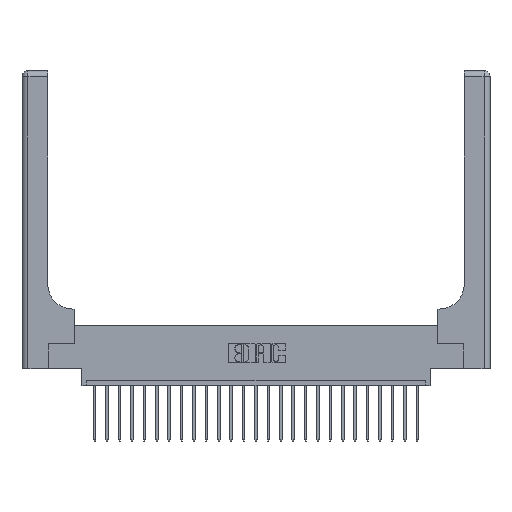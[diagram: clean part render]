
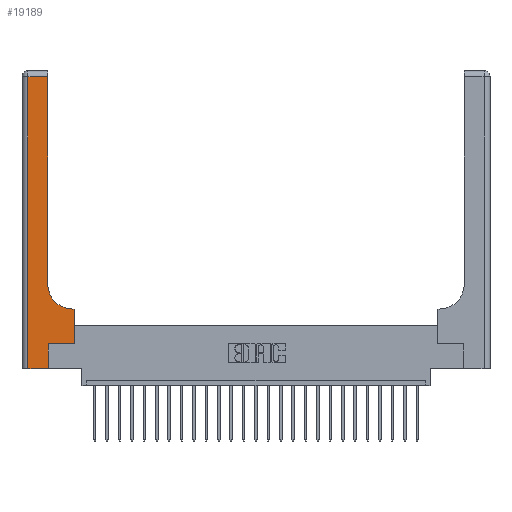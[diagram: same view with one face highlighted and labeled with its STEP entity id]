
A CAD part, top view. The second image highlights one B-rep face of the part: STEP entity #19189.
In plain terms, the highlighted planar face has unit normal (0, 0, 1).
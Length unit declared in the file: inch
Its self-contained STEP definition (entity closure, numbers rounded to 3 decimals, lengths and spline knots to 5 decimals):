
#389 = VERTEX_POINT ( 'NONE', #19670 ) ;
#482 = ORIENTED_EDGE ( 'NONE', *, *, #1757, .T. ) ;
#861 = AXIS2_PLACEMENT_3D ( 'NONE', #8938, #9064, #5103 ) ;
#1435 = DIRECTION ( 'NONE',  ( 1., 0., 0. ) ) ;
#1757 = EDGE_CURVE ( 'NONE', #12092, #18439, #12728, .T. ) ;
#1889 = CARTESIAN_POINT ( 'NONE',  ( 0.265, 0.25, 0.37 ) ) ;
#2095 = EDGE_CURVE ( 'NONE', #8628, #21289, #4739, .T. ) ;
#2150 = CARTESIAN_POINT ( 'NONE',  ( 0.528, 0.25, 0.37 ) ) ;
#2192 = AXIS2_PLACEMENT_3D ( 'NONE', #3518, #24505, #9337 ) ;
#2385 = ORIENTED_EDGE ( 'NONE', *, *, #19223, .T. ) ;
#3319 = CARTESIAN_POINT ( 'NONE',  ( 0.265, 0., 0.37 ) ) ;
#3518 = CARTESIAN_POINT ( 'NONE',  ( 0., 3., 0.37 ) ) ;
#3534 = CARTESIAN_POINT ( 'NONE',  ( 0.26, 3., 0.37 ) ) ;
#3911 = ORIENTED_EDGE ( 'NONE', *, *, #13607, .T. ) ;
#4010 = VECTOR ( 'NONE', #9216, 39.37008 ) ;
#4739 = LINE ( 'NONE', #19775, #7681 ) ;
#4780 = VERTEX_POINT ( 'NONE', #6330 ) ;
#4999 = CARTESIAN_POINT ( 'NONE',  ( 0.528, 0.6, 0.37 ) ) ;
#5056 = ORIENTED_EDGE ( 'NONE', *, *, #9811, .T. ) ;
#5103 = DIRECTION ( 'NONE',  ( 1., 0., 0. ) ) ;
#5195 = LINE ( 'NONE', #18601, #22614 ) ;
#5197 = CIRCLE ( 'NONE', #861, 0.25 ) ;
#6090 = VECTOR ( 'NONE', #1435, 39.37008 ) ;
#6330 = CARTESIAN_POINT ( 'NONE',  ( 0.06, 2.94, 0.37 ) ) ;
#6669 = VERTEX_POINT ( 'NONE', #23704 ) ;
#7644 = VECTOR ( 'NONE', #9662, 39.37008 ) ;
#7681 = VECTOR ( 'NONE', #16159, 39.37008 ) ;
#7835 = LINE ( 'NONE', #1889, #8674 ) ;
#8048 = ORIENTED_EDGE ( 'NONE', *, *, #12632, .T. ) ;
#8352 = DIRECTION ( 'NONE',  ( -1., 0., 0. ) ) ;
#8628 = VERTEX_POINT ( 'NONE', #4999 ) ;
#8674 = VECTOR ( 'NONE', #19263, 39.37008 ) ;
#8938 = CARTESIAN_POINT ( 'NONE',  ( 0.51, 0.85, 0.37 ) ) ;
#9064 = DIRECTION ( 'NONE',  ( 0., 0., -1. ) ) ;
#9204 = CARTESIAN_POINT ( 'NONE',  ( 0.06, 3., 0.37 ) ) ;
#9216 = DIRECTION ( 'NONE',  ( 0., 1., 0. ) ) ;
#9251 = ORIENTED_EDGE ( 'NONE', *, *, #14322, .T. ) ;
#9337 = DIRECTION ( 'NONE',  ( -1., 0., 0. ) ) ;
#9470 = LINE ( 'NONE', #9204, #11715 ) ;
#9662 = DIRECTION ( 'NONE',  ( 0., 1., 0. ) ) ;
#9811 = EDGE_CURVE ( 'NONE', #6669, #13739, #7835, .T. ) ;
#10947 = PLANE ( 'NONE',  #2192 ) ;
#11275 = LINE ( 'NONE', #16980, #7644 ) ;
#11715 = VECTOR ( 'NONE', #24123, 39.37008 ) ;
#12092 = VERTEX_POINT ( 'NONE', #13846 ) ;
#12632 = EDGE_CURVE ( 'NONE', #13739, #8628, #5195, .T. ) ;
#12728 = LINE ( 'NONE', #18435, #6090 ) ;
#13600 = CARTESIAN_POINT ( 'NONE',  ( 0.26, 0.85, 0.37 ) ) ;
#13607 = EDGE_CURVE ( 'NONE', #24260, #389, #20541, .T. ) ;
#13739 = VERTEX_POINT ( 'NONE', #2150 ) ;
#13846 = CARTESIAN_POINT ( 'NONE',  ( 0.06, 0., 0.37 ) ) ;
#13934 = ORIENTED_EDGE ( 'NONE', *, *, #17517, .T. ) ;
#14322 = EDGE_CURVE ( 'NONE', #21289, #24260, #5197, .T. ) ;
#14892 = EDGE_CURVE ( 'NONE', #18439, #6669, #11275, .T. ) ;
#16159 = DIRECTION ( 'NONE',  ( -1., 0., 0. ) ) ;
#16249 = CARTESIAN_POINT ( 'NONE',  ( 0.51, 0.6, 0.37 ) ) ;
#16505 = ORIENTED_EDGE ( 'NONE', *, *, #14892, .T. ) ;
#16980 = CARTESIAN_POINT ( 'NONE',  ( 0.265, 0., 0.37 ) ) ;
#17517 = EDGE_CURVE ( 'NONE', #389, #4780, #17909, .T. ) ;
#17909 = LINE ( 'NONE', #20264, #23932 ) ;
#18435 = CARTESIAN_POINT ( 'NONE',  ( 0., 0., 0.37 ) ) ;
#18439 = VERTEX_POINT ( 'NONE', #3319 ) ;
#18601 = CARTESIAN_POINT ( 'NONE',  ( 0.528, 0.25, 0.37 ) ) ;
#19025 = FACE_OUTER_BOUND ( 'NONE', #23286, .T. ) ;
#19189 = ADVANCED_FACE ( 'NONE', ( #19025 ), #10947, .F. ) ;
#19223 = EDGE_CURVE ( 'NONE', #4780, #12092, #9470, .T. ) ;
#19263 = DIRECTION ( 'NONE',  ( 1., 0., 0. ) ) ;
#19670 = CARTESIAN_POINT ( 'NONE',  ( 0.26, 2.94, 0.37 ) ) ;
#19775 = CARTESIAN_POINT ( 'NONE',  ( 0.26, 0.6, 0.37 ) ) ;
#20264 = CARTESIAN_POINT ( 'NONE',  ( 0., 2.94, 0.37 ) ) ;
#20541 = LINE ( 'NONE', #3534, #4010 ) ;
#21289 = VERTEX_POINT ( 'NONE', #16249 ) ;
#21536 = ORIENTED_EDGE ( 'NONE', *, *, #2095, .T. ) ;
#22099 = DIRECTION ( 'NONE',  ( 0., 1., 0. ) ) ;
#22614 = VECTOR ( 'NONE', #22099, 39.37008 ) ;
#23286 = EDGE_LOOP ( 'NONE', ( #3911, #13934, #2385, #482, #16505, #5056, #8048, #21536, #9251 ) ) ;
#23704 = CARTESIAN_POINT ( 'NONE',  ( 0.265, 0.25, 0.37 ) ) ;
#23932 = VECTOR ( 'NONE', #8352, 39.37008 ) ;
#24123 = DIRECTION ( 'NONE',  ( 0., -1., 0. ) ) ;
#24260 = VERTEX_POINT ( 'NONE', #13600 ) ;
#24505 = DIRECTION ( 'NONE',  ( 0., 0., -1. ) ) ;
